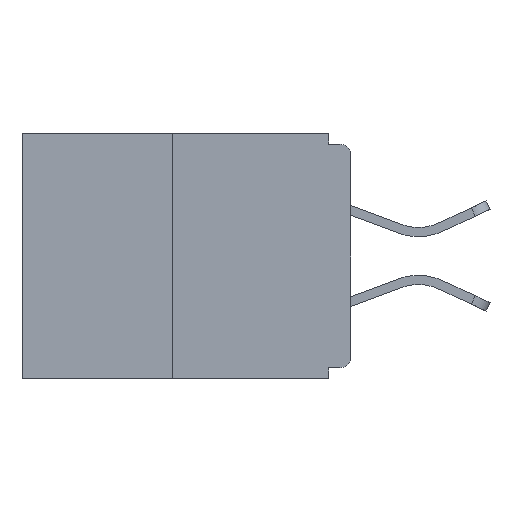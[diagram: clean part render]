
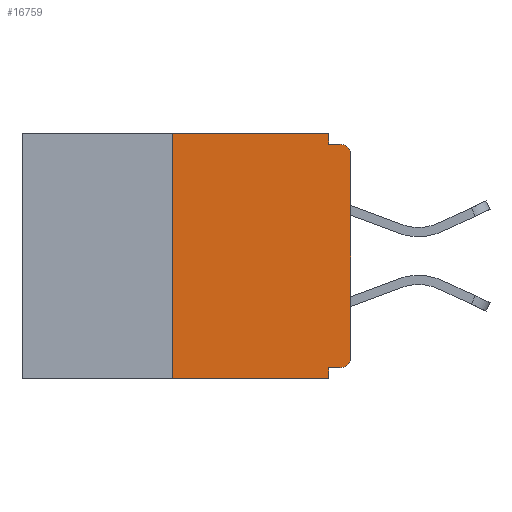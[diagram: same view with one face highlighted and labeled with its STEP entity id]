
A CAD part, left-side view. The second image highlights one B-rep face of the part: STEP entity #16759.
In plain terms, the highlighted planar face has unit normal (-1, 0, 0).
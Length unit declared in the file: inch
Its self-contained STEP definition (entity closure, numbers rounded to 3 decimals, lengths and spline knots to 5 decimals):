
#475 = VERTEX_POINT ( 'NONE', #3040 ) ;
#644 = ORIENTED_EDGE ( 'NONE', *, *, #6944, .T. ) ;
#824 = CARTESIAN_POINT ( 'NONE',  ( 0., 0.46, -0.343 ) ) ;
#911 = CARTESIAN_POINT ( 'NONE',  ( 0., 0., 0. ) ) ;
#1184 = VERTEX_POINT ( 'NONE', #11872 ) ;
#1269 = DIRECTION ( 'NONE',  ( 0., 1., 0. ) ) ;
#1391 = LINE ( 'NONE', #4784, #2216 ) ;
#2216 = VECTOR ( 'NONE', #15319, 39.37008 ) ;
#2490 = VECTOR ( 'NONE', #3820, 39.37008 ) ;
#2514 = EDGE_LOOP ( 'NONE', ( #16733, #14055, #9783, #3665, #9441, #5401, #644, #12440, #11994, #4474 ) ) ;
#2631 = CARTESIAN_POINT ( 'NONE',  ( 0., 0.031, 0. ) ) ;
#3040 = CARTESIAN_POINT ( 'NONE',  ( 0., 0.031, -0.328 ) ) ;
#3140 = DIRECTION ( 'NONE',  ( 0., 0., -1. ) ) ;
#3147 = EDGE_CURVE ( 'NONE', #17188, #16563, #3891, .T. ) ;
#3334 = CARTESIAN_POINT ( 'NONE',  ( 0., 0.25, 0. ) ) ;
#3413 = EDGE_CURVE ( 'NONE', #19218, #16772, #20114, .T. ) ;
#3509 = AXIS2_PLACEMENT_3D ( 'NONE', #7085, #5426, #3910 ) ;
#3665 = ORIENTED_EDGE ( 'NONE', *, *, #6468, .F. ) ;
#3700 = VECTOR ( 'NONE', #16233, 39.37008 ) ;
#3820 = DIRECTION ( 'NONE',  ( 0., -1., 0. ) ) ;
#3826 = DIRECTION ( 'NONE',  ( 0., -1., 0. ) ) ;
#3891 = LINE ( 'NONE', #16428, #3700 ) ;
#3910 = DIRECTION ( 'NONE',  ( 0., 0., -1. ) ) ;
#3945 = CARTESIAN_POINT ( 'NONE',  ( 0., 0.46, 0. ) ) ;
#4045 = CARTESIAN_POINT ( 'NONE',  ( 0., 0.46, 0. ) ) ;
#4240 = LINE ( 'NONE', #3945, #13275 ) ;
#4343 = FACE_OUTER_BOUND ( 'NONE', #2514, .T. ) ;
#4474 = ORIENTED_EDGE ( 'NONE', *, *, #7877, .F. ) ;
#4483 = CARTESIAN_POINT ( 'NONE',  ( 0., 0.015, -0.03 ) ) ;
#4735 = AXIS2_PLACEMENT_3D ( 'NONE', #4483, #16840, #3140 ) ;
#4784 = CARTESIAN_POINT ( 'NONE',  ( 0., 0.031, 0. ) ) ;
#5321 = LINE ( 'NONE', #824, #2490 ) ;
#5401 = ORIENTED_EDGE ( 'NONE', *, *, #3413, .T. ) ;
#5426 = DIRECTION ( 'NONE',  ( -1., 0., 0. ) ) ;
#5701 = DIRECTION ( 'NONE',  ( 0., 0., 1. ) ) ;
#6468 = EDGE_CURVE ( 'NONE', #475, #14563, #10477, .T. ) ;
#6944 = EDGE_CURVE ( 'NONE', #16772, #1184, #7278, .T. ) ;
#7015 = EDGE_CURVE ( 'NONE', #1184, #12380, #13561, .T. ) ;
#7085 = CARTESIAN_POINT ( 'NONE',  ( 0., 0.015, -0.313 ) ) ;
#7278 = LINE ( 'NONE', #911, #10962 ) ;
#7528 = CARTESIAN_POINT ( 'NONE',  ( 0., 0.015, -0.015 ) ) ;
#7693 = CARTESIAN_POINT ( 'NONE',  ( 0., 0.031, -0.343 ) ) ;
#7877 = EDGE_CURVE ( 'NONE', #16749, #15430, #1391, .T. ) ;
#8053 = VECTOR ( 'NONE', #1269, 39.37008 ) ;
#8670 = VECTOR ( 'NONE', #10378, 39.37008 ) ;
#8771 = CARTESIAN_POINT ( 'NONE',  ( 0., 0.25, -0.343 ) ) ;
#9007 = EDGE_CURVE ( 'NONE', #17188, #14563, #5321, .T. ) ;
#9441 = ORIENTED_EDGE ( 'NONE', *, *, #13299, .F. ) ;
#9783 = ORIENTED_EDGE ( 'NONE', *, *, #9007, .T. ) ;
#9942 = VECTOR ( 'NONE', #3826, 39.37008 ) ;
#10378 = DIRECTION ( 'NONE',  ( 0., 0., -1. ) ) ;
#10459 = AXIS2_PLACEMENT_3D ( 'NONE', #4045, #10618, #10518 ) ;
#10477 = LINE ( 'NONE', #13618, #8670 ) ;
#10518 = DIRECTION ( 'NONE',  ( 0., 0., -1. ) ) ;
#10618 = DIRECTION ( 'NONE',  ( 1., 0., 0. ) ) ;
#10765 = CARTESIAN_POINT ( 'NONE',  ( 0., 0.015, -0.328 ) ) ;
#10962 = VECTOR ( 'NONE', #5701, 39.37008 ) ;
#11524 = EDGE_CURVE ( 'NONE', #15430, #12380, #11602, .T. ) ;
#11602 = LINE ( 'NONE', #17785, #9942 ) ;
#11738 = DIRECTION ( 'NONE',  ( 0., -1., 0. ) ) ;
#11872 = CARTESIAN_POINT ( 'NONE',  ( 0., 0., -0.03 ) ) ;
#11994 = ORIENTED_EDGE ( 'NONE', *, *, #11524, .F. ) ;
#12227 = LINE ( 'NONE', #15282, #8053 ) ;
#12233 = CARTESIAN_POINT ( 'NONE',  ( 0., 0., -0.313 ) ) ;
#12380 = VERTEX_POINT ( 'NONE', #7528 ) ;
#12440 = ORIENTED_EDGE ( 'NONE', *, *, #7015, .T. ) ;
#13275 = VECTOR ( 'NONE', #11738, 39.37008 ) ;
#13299 = EDGE_CURVE ( 'NONE', #19218, #475, #12227, .T. ) ;
#13561 = CIRCLE ( 'NONE', #4735, 0.015 ) ;
#13618 = CARTESIAN_POINT ( 'NONE',  ( 0., 0.031, -0.343 ) ) ;
#14055 = ORIENTED_EDGE ( 'NONE', *, *, #3147, .F. ) ;
#14563 = VERTEX_POINT ( 'NONE', #7693 ) ;
#15282 = CARTESIAN_POINT ( 'NONE',  ( 0., 0., -0.328 ) ) ;
#15319 = DIRECTION ( 'NONE',  ( 0., 0., -1. ) ) ;
#15361 = CARTESIAN_POINT ( 'NONE',  ( 0., 0.031, -0.015 ) ) ;
#15430 = VERTEX_POINT ( 'NONE', #15361 ) ;
#16233 = DIRECTION ( 'NONE',  ( 0., 0., 1. ) ) ;
#16428 = CARTESIAN_POINT ( 'NONE',  ( 0., 0.25, 0. ) ) ;
#16563 = VERTEX_POINT ( 'NONE', #3334 ) ;
#16733 = ORIENTED_EDGE ( 'NONE', *, *, #18856, .F. ) ;
#16749 = VERTEX_POINT ( 'NONE', #2631 ) ;
#16759 = ADVANCED_FACE ( 'NONE', ( #4343 ), #18123, .F. ) ;
#16772 = VERTEX_POINT ( 'NONE', #12233 ) ;
#16840 = DIRECTION ( 'NONE',  ( -1., 0., 0. ) ) ;
#17188 = VERTEX_POINT ( 'NONE', #8771 ) ;
#17785 = CARTESIAN_POINT ( 'NONE',  ( 0., 0., -0.015 ) ) ;
#18123 = PLANE ( 'NONE',  #10459 ) ;
#18856 = EDGE_CURVE ( 'NONE', #16563, #16749, #4240, .T. ) ;
#19218 = VERTEX_POINT ( 'NONE', #10765 ) ;
#20114 = CIRCLE ( 'NONE', #3509, 0.015 ) ;
